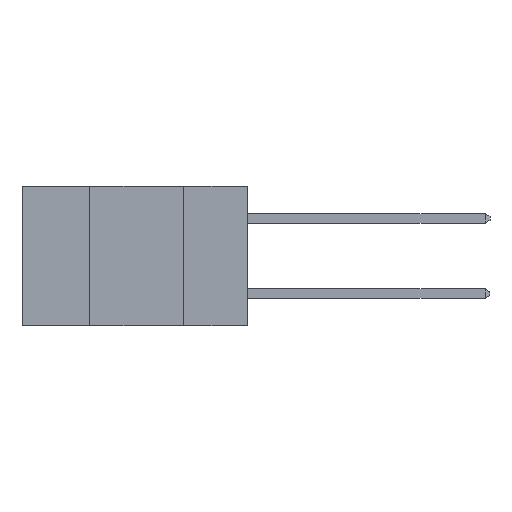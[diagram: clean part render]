
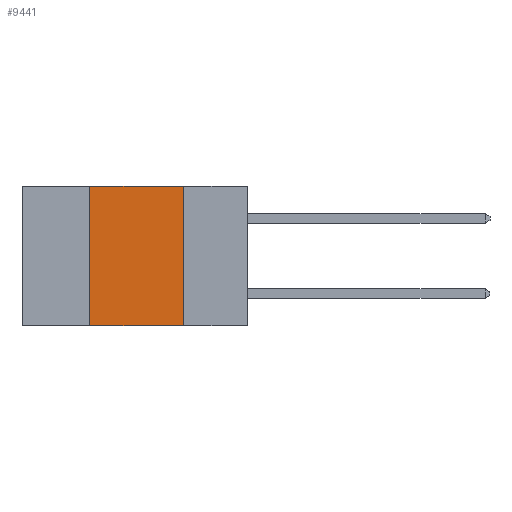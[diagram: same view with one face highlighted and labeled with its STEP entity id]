
A CAD part, left-side view. The second image highlights one B-rep face of the part: STEP entity #9441.
In plain terms, the highlighted planar face has unit normal (-1, 0, 0).
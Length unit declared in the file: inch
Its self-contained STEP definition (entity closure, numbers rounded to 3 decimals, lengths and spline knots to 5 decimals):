
#59 = VERTEX_POINT ( 'NONE', #74 ) ;
#74 = CARTESIAN_POINT ( 'NONE',  ( 0., 0.42, -0.37 ) ) ;
#546 = LINE ( 'NONE', #7408, #3469 ) ;
#1380 = EDGE_CURVE ( 'NONE', #59, #7384, #7232, .T. ) ;
#1667 = LINE ( 'NONE', #6679, #9051 ) ;
#2332 = EDGE_CURVE ( 'NONE', #14067, #10688, #3476, .T. ) ;
#3469 = VECTOR ( 'NONE', #15536, 39.37008 ) ;
#3476 = LINE ( 'NONE', #4452, #6766 ) ;
#4452 = CARTESIAN_POINT ( 'NONE',  ( 0., 0.17, 0. ) ) ;
#5399 = FACE_OUTER_BOUND ( 'NONE', #6944, .T. ) ;
#6283 = CARTESIAN_POINT ( 'NONE',  ( 0., 0.17, 0. ) ) ;
#6679 = CARTESIAN_POINT ( 'NONE',  ( 0., 0.6, -0.37 ) ) ;
#6766 = VECTOR ( 'NONE', #11394, 39.37008 ) ;
#6944 = EDGE_LOOP ( 'NONE', ( #14012, #14159, #14340, #15042 ) ) ;
#7232 = LINE ( 'NONE', #15094, #14462 ) ;
#7384 = VERTEX_POINT ( 'NONE', #16659 ) ;
#7408 = CARTESIAN_POINT ( 'NONE',  ( 0., 0.6, 0. ) ) ;
#7923 = DIRECTION ( 'NONE',  ( 1., 0., 0. ) ) ;
#9051 = VECTOR ( 'NONE', #16159, 39.37008 ) ;
#9441 = ADVANCED_FACE ( 'NONE', ( #5399 ), #14729, .F. ) ;
#10688 = VERTEX_POINT ( 'NONE', #17194 ) ;
#11394 = DIRECTION ( 'NONE',  ( 0., 0., -1. ) ) ;
#11818 = AXIS2_PLACEMENT_3D ( 'NONE', #13389, #7923, #17344 ) ;
#13389 = CARTESIAN_POINT ( 'NONE',  ( 0., 0.6, 0. ) ) ;
#14012 = ORIENTED_EDGE ( 'NONE', *, *, #2332, .F. ) ;
#14067 = VERTEX_POINT ( 'NONE', #6283 ) ;
#14159 = ORIENTED_EDGE ( 'NONE', *, *, #15464, .F. ) ;
#14340 = ORIENTED_EDGE ( 'NONE', *, *, #1380, .F. ) ;
#14462 = VECTOR ( 'NONE', #17525, 39.37008 ) ;
#14729 = PLANE ( 'NONE',  #11818 ) ;
#15042 = ORIENTED_EDGE ( 'NONE', *, *, #16444, .T. ) ;
#15094 = CARTESIAN_POINT ( 'NONE',  ( 0., 0.42, 0. ) ) ;
#15464 = EDGE_CURVE ( 'NONE', #7384, #14067, #546, .T. ) ;
#15536 = DIRECTION ( 'NONE',  ( 0., -1., 0. ) ) ;
#16159 = DIRECTION ( 'NONE',  ( 0., -1., 0. ) ) ;
#16444 = EDGE_CURVE ( 'NONE', #59, #10688, #1667, .T. ) ;
#16659 = CARTESIAN_POINT ( 'NONE',  ( 0., 0.42, 0. ) ) ;
#17194 = CARTESIAN_POINT ( 'NONE',  ( 0., 0.17, -0.37 ) ) ;
#17344 = DIRECTION ( 'NONE',  ( 0., 0., -1. ) ) ;
#17525 = DIRECTION ( 'NONE',  ( 0., 0., 1. ) ) ;
